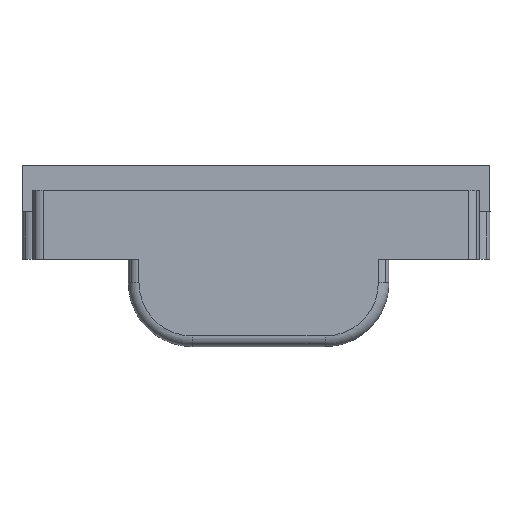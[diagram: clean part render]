
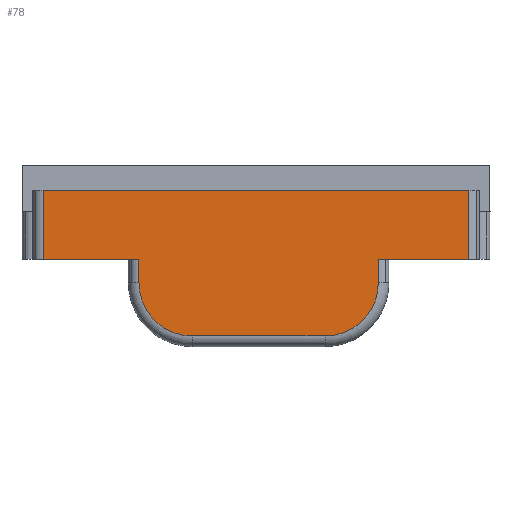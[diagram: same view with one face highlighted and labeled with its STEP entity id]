
A CAD part, front view. The second image highlights one B-rep face of the part: STEP entity #78.
In plain terms, the highlighted planar face has unit normal (0, -1, 0).
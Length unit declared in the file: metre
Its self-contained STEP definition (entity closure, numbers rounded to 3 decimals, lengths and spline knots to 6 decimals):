
#78=ADVANCED_FACE('0:64550',(#184),#185,.T.);
#184=FACE_OUTER_BOUND('',#344,.T.);
#185=PLANE('',#345);
#344=EDGE_LOOP('',(#645,#646,#647,#648,#649,#650,#651,#652,#653,#654));
#345=AXIS2_PLACEMENT_3D('',#655,#656,#657);
#645=ORIENTED_EDGE('',*,*,#1205,.F.);
#646=ORIENTED_EDGE('',*,*,#1188,.F.);
#647=ORIENTED_EDGE('',*,*,#1202,.F.);
#648=ORIENTED_EDGE('',*,*,#1198,.F.);
#649=ORIENTED_EDGE('',*,*,#1197,.F.);
#650=ORIENTED_EDGE('',*,*,#1184,.F.);
#651=ORIENTED_EDGE('',*,*,#1206,.F.);
#652=ORIENTED_EDGE('',*,*,#1140,.F.);
#653=ORIENTED_EDGE('',*,*,#1207,.F.);
#654=ORIENTED_EDGE('',*,*,#1208,.F.);
#655=CARTESIAN_POINT('',(-0.082,0.002093,-0.0223));
#656=DIRECTION('',(0.0,-1.0,0.0));
#657=DIRECTION('',(0.0,0.0,-1.0));
#1140=EDGE_CURVE('0:64748',#1387,#1389,#1390,.T.);
#1184=EDGE_CURVE('0:64742',#1474,#1476,#1477,.T.);
#1188=EDGE_CURVE('0:64736',#1482,#1484,#1485,.T.);
#1197=EDGE_CURVE('0:64709',#1476,#1494,#1498,.T.);
#1198=EDGE_CURVE('0:64718',#1494,#1499,#1500,.T.);
#1202=EDGE_CURVE('0:64727',#1499,#1482,#1505,.T.);
#1205=EDGE_CURVE('0:64739',#1484,#1509,#1510,.T.);
#1206=EDGE_CURVE('0:64745',#1389,#1474,#1511,.T.);
#1207=EDGE_CURVE('0:64751',#1512,#1387,#1513,.F.);
#1208=EDGE_CURVE('0:64754',#1509,#1512,#1514,.T.);
#1387=VERTEX_POINT('',#1752);
#1389=VERTEX_POINT('',#1754);
#1390=LINE('',#1755,#1756);
#1474=VERTEX_POINT('',#1861);
#1476=VERTEX_POINT('',#1863);
#1477=LINE('',#1864,#1865);
#1482=VERTEX_POINT('',#1871);
#1484=VERTEX_POINT('',#1873);
#1485=LINE('',#1874,#1875);
#1494=VERTEX_POINT('',#1886);
#1498=CIRCLE('',#1890,0.005);
#1499=VERTEX_POINT('',#1891);
#1500=LINE('',#1892,#1893);
#1505=CIRCLE('',#1898,0.005);
#1509=VERTEX_POINT('',#1903);
#1510=LINE('',#1904,#1905);
#1511=LINE('',#1906,#1907);
#1512=VERTEX_POINT('',#1908);
#1513=LINE('',#1909,#1910);
#1514=LINE('',#1911,#1912);
#1752=CARTESIAN_POINT('',(-0.069,0.002093,-0.0251));
#1754=CARTESIAN_POINT('',(-0.069,0.002093,-0.0316));
#1755=CARTESIAN_POINT('',(-0.069,0.002093,-0.0301));
#1756=VECTOR('',#2194,0.0065);
#1861=CARTESIAN_POINT('',(-0.0775,0.002093,-0.0316));
#1863=CARTESIAN_POINT('',(-0.0775,0.002093,-0.0338));
#1864=CARTESIAN_POINT('',(-0.0775,0.002093,-0.02295));
#1865=VECTOR('',#2282,0.0022);
#1871=CARTESIAN_POINT('',(-0.1,0.002093,-0.0338));
#1873=CARTESIAN_POINT('',(-0.1,0.002093,-0.0316));
#1874=CARTESIAN_POINT('',(-0.1,0.002093,-0.022529));
#1875=VECTOR('',#2290,0.0022);
#1886=CARTESIAN_POINT('',(-0.0825,0.002093,-0.0388));
#1890=AXIS2_PLACEMENT_3D('',#2311,#2312,#2313);
#1891=CARTESIAN_POINT('',(-0.095,0.002093,-0.0388));
#1892=CARTESIAN_POINT('',(-0.092,0.002093,-0.0388));
#1893=VECTOR('',#2314,0.0125);
#1898=AXIS2_PLACEMENT_3D('',#2324,#2325,#2326);
#1903=CARTESIAN_POINT('',(-0.109,0.002093,-0.0316));
#1904=CARTESIAN_POINT('',(-0.0975,0.002093,-0.0316));
#1905=VECTOR('',#2331,0.009);
#1906=CARTESIAN_POINT('',(-0.0915,0.002093,-0.0316));
#1907=VECTOR('',#2332,0.0085);
#1908=CARTESIAN_POINT('',(-0.109,0.002093,-0.0251));
#1909=CARTESIAN_POINT('',(-0.086,0.002093,-0.0251));
#1910=VECTOR('',#2333,0.04);
#1911=CARTESIAN_POINT('',(-0.109,0.002093,-0.0301));
#1912=VECTOR('',#2334,0.0065);
#2194=DIRECTION('',(0.0,0.0,-1.0));
#2282=DIRECTION('',(0.0,0.0,-1.0));
#2290=DIRECTION('',(0.0,0.0,1.0));
#2311=CARTESIAN_POINT('',(-0.0825,0.002093,-0.0338));
#2312=DIRECTION('',(0.0,1.0,0.0));
#2313=DIRECTION('',(0.473,0.0,-0.881));
#2314=DIRECTION('',(-1.0,0.0,0.0));
#2324=CARTESIAN_POINT('',(-0.095,0.002093,-0.0338));
#2325=DIRECTION('',(0.0,1.0,0.0));
#2326=DIRECTION('',(-0.707,0.0,-0.707));
#2331=DIRECTION('',(-1.0,0.0,0.0));
#2332=DIRECTION('',(-1.0,0.0,0.0));
#2333=DIRECTION('',(-1.0,0.0,0.0));
#2334=DIRECTION('',(0.0,0.0,1.0));
